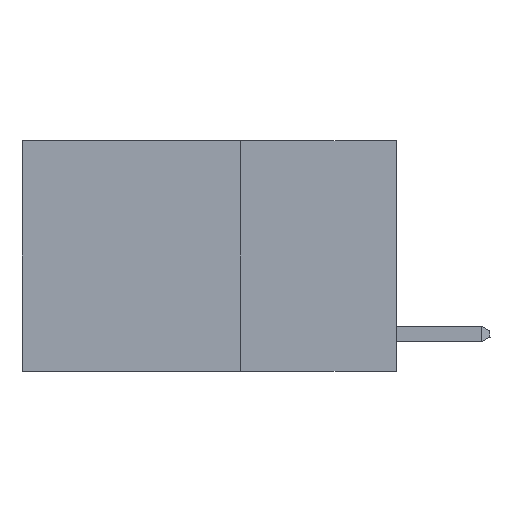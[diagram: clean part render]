
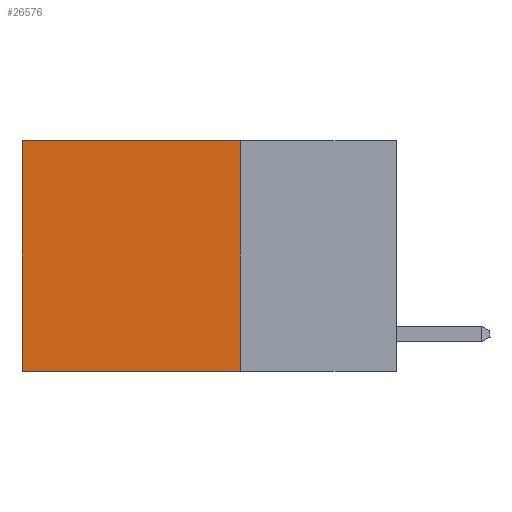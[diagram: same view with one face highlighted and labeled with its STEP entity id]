
A CAD part, left-side view. The second image highlights one B-rep face of the part: STEP entity #26576.
In plain terms, the highlighted planar face has unit normal (-1, 0, 0).
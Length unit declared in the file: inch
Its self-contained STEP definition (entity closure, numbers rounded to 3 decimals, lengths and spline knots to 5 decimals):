
#2600 = EDGE_CURVE ( 'NONE', #2891, #6471, #16353, .T. ) ;
#2891 = VERTEX_POINT ( 'NONE', #15970 ) ;
#3234 = AXIS2_PLACEMENT_3D ( 'NONE', #24130, #17876, #5084 ) ;
#4357 = VECTOR ( 'NONE', #21559, 39.37008 ) ;
#4690 = CARTESIAN_POINT ( 'NONE',  ( 0.2625, 0.25, -0.37 ) ) ;
#4979 = ORIENTED_EDGE ( 'NONE', *, *, #6933, .F. ) ;
#5084 = DIRECTION ( 'NONE',  ( 0., 0., -1. ) ) ;
#5828 = LINE ( 'NONE', #6898, #11475 ) ;
#6431 = DIRECTION ( 'NONE',  ( 0., 0., -1. ) ) ;
#6471 = VERTEX_POINT ( 'NONE', #9247 ) ;
#6534 = VECTOR ( 'NONE', #11096, 39.37008 ) ;
#6898 = CARTESIAN_POINT ( 'NONE',  ( 0.2625, 0.6, 0. ) ) ;
#6933 = EDGE_CURVE ( 'NONE', #2891, #8553, #25681, .T. ) ;
#8553 = VERTEX_POINT ( 'NONE', #16125 ) ;
#9247 = CARTESIAN_POINT ( 'NONE',  ( 0.2625, 0.6, 0. ) ) ;
#10712 = CARTESIAN_POINT ( 'NONE',  ( 0.2625, 0.25, 0. ) ) ;
#10930 = CARTESIAN_POINT ( 'NONE',  ( 0.2625, 0.25, 0. ) ) ;
#11096 = DIRECTION ( 'NONE',  ( 0., 1., 0. ) ) ;
#11475 = VECTOR ( 'NONE', #21799, 39.37008 ) ;
#15970 = CARTESIAN_POINT ( 'NONE',  ( 0.2625, 0.25, 0. ) ) ;
#16125 = CARTESIAN_POINT ( 'NONE',  ( 0.2625, 0.25, -0.37 ) ) ;
#16353 = LINE ( 'NONE', #10930, #4357 ) ;
#16847 = EDGE_LOOP ( 'NONE', ( #18594, #27048, #4979, #21809 ) ) ;
#17876 = DIRECTION ( 'NONE',  ( 1., 0., 0. ) ) ;
#18594 = ORIENTED_EDGE ( 'NONE', *, *, #27134, .T. ) ;
#19920 = PLANE ( 'NONE',  #3234 ) ;
#20754 = VECTOR ( 'NONE', #6431, 39.37008 ) ;
#20819 = FACE_OUTER_BOUND ( 'NONE', #16847, .T. ) ;
#21559 = DIRECTION ( 'NONE',  ( 0., 1., 0. ) ) ;
#21799 = DIRECTION ( 'NONE',  ( 0., 0., -1. ) ) ;
#21809 = ORIENTED_EDGE ( 'NONE', *, *, #2600, .T. ) ;
#23518 = CARTESIAN_POINT ( 'NONE',  ( 0.2625, 0.6, -0.37 ) ) ;
#23705 = EDGE_CURVE ( 'NONE', #8553, #24783, #24177, .T. ) ;
#24130 = CARTESIAN_POINT ( 'NONE',  ( 0.2625, 0.25, 0. ) ) ;
#24177 = LINE ( 'NONE', #4690, #6534 ) ;
#24783 = VERTEX_POINT ( 'NONE', #23518 ) ;
#25681 = LINE ( 'NONE', #10712, #20754 ) ;
#26576 = ADVANCED_FACE ( 'NONE', ( #20819 ), #19920, .F. ) ;
#27048 = ORIENTED_EDGE ( 'NONE', *, *, #23705, .F. ) ;
#27134 = EDGE_CURVE ( 'NONE', #6471, #24783, #5828, .T. ) ;
